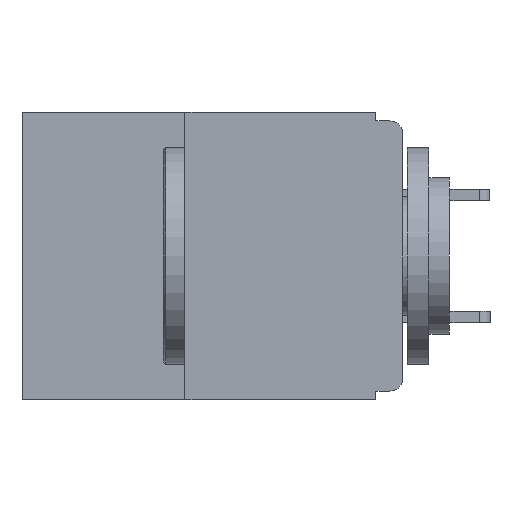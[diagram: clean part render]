
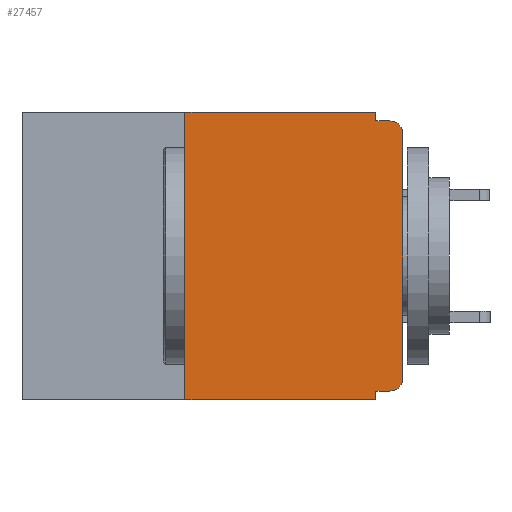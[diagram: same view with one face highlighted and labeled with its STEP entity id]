
A CAD part, left-side view. The second image highlights one B-rep face of the part: STEP entity #27457.
In plain terms, the highlighted planar face has unit normal (-1, 0, 0).
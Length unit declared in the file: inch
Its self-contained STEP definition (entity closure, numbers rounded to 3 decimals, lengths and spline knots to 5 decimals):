
#1856 = ORIENTED_EDGE ( 'NONE', *, *, #5926, .F. ) ;
#2237 = LINE ( 'NONE', #5492, #8270 ) ;
#2534 = CARTESIAN_POINT ( 'NONE',  ( 0., 0.031, -0.33 ) ) ;
#2595 = ORIENTED_EDGE ( 'NONE', *, *, #11031, .F. ) ;
#3029 = ORIENTED_EDGE ( 'NONE', *, *, #3732, .T. ) ;
#3189 = CIRCLE ( 'NONE', #19595, 0.015 ) ;
#3732 = EDGE_CURVE ( 'NONE', #11708, #23164, #3189, .T. ) ;
#4182 = VECTOR ( 'NONE', #6975, 39.37008 ) ;
#5186 = EDGE_CURVE ( 'NONE', #17108, #11934, #23696, .T. ) ;
#5492 = CARTESIAN_POINT ( 'NONE',  ( 0., 0.437, -0.33 ) ) ;
#5926 = EDGE_CURVE ( 'NONE', #29202, #24118, #17416, .T. ) ;
#6591 = PLANE ( 'NONE',  #20163 ) ;
#6975 = DIRECTION ( 'NONE',  ( 0., 0., -1. ) ) ;
#7290 = VERTEX_POINT ( 'NONE', #11916 ) ;
#7435 = EDGE_CURVE ( 'NONE', #14419, #11934, #23615, .T. ) ;
#7765 = CARTESIAN_POINT ( 'NONE',  ( 0., 0., -0.01 ) ) ;
#7867 = DIRECTION ( 'NONE',  ( 0., -1., 0. ) ) ;
#7897 = VERTEX_POINT ( 'NONE', #8672 ) ;
#8225 = ORIENTED_EDGE ( 'NONE', *, *, #27355, .F. ) ;
#8270 = VECTOR ( 'NONE', #14558, 39.37008 ) ;
#8415 = ORIENTED_EDGE ( 'NONE', *, *, #14493, .T. ) ;
#8672 = CARTESIAN_POINT ( 'NONE',  ( 0., 0.25, -0.33 ) ) ;
#8849 = DIRECTION ( 'NONE',  ( 1., 0., 0. ) ) ;
#9213 = CARTESIAN_POINT ( 'NONE',  ( 0., 0.031, 0. ) ) ;
#9583 = ORIENTED_EDGE ( 'NONE', *, *, #5186, .T. ) ;
#10582 = ORIENTED_EDGE ( 'NONE', *, *, #24138, .T. ) ;
#10684 = CARTESIAN_POINT ( 'NONE',  ( 0., 0., -0.32 ) ) ;
#10796 = DIRECTION ( 'NONE',  ( 0., 0., 1. ) ) ;
#11031 = EDGE_CURVE ( 'NONE', #11708, #29202, #25164, .T. ) ;
#11708 = VERTEX_POINT ( 'NONE', #15775 ) ;
#11916 = CARTESIAN_POINT ( 'NONE',  ( 0., 0.25, 0. ) ) ;
#11934 = VERTEX_POINT ( 'NONE', #27694 ) ;
#11983 = LINE ( 'NONE', #27381, #28444 ) ;
#12973 = DIRECTION ( 'NONE',  ( 0., 1., 0. ) ) ;
#13116 = CARTESIAN_POINT ( 'NONE',  ( 0., 0., -0.025 ) ) ;
#13993 = ORIENTED_EDGE ( 'NONE', *, *, #18505, .F. ) ;
#14419 = VERTEX_POINT ( 'NONE', #25546 ) ;
#14493 = EDGE_CURVE ( 'NONE', #7897, #24118, #2237, .T. ) ;
#14558 = DIRECTION ( 'NONE',  ( 0., -1., 0. ) ) ;
#15058 = FACE_OUTER_BOUND ( 'NONE', #21268, .T. ) ;
#15775 = CARTESIAN_POINT ( 'NONE',  ( 0., 0.015, -0.32 ) ) ;
#17108 = VERTEX_POINT ( 'NONE', #13116 ) ;
#17137 = VECTOR ( 'NONE', #12973, 39.37008 ) ;
#17209 = VECTOR ( 'NONE', #10796, 39.37008 ) ;
#17416 = LINE ( 'NONE', #21441, #24051 ) ;
#17811 = CARTESIAN_POINT ( 'NONE',  ( 0., 0.031, -0.32 ) ) ;
#18505 = EDGE_CURVE ( 'NONE', #7290, #25681, #21759, .T. ) ;
#19595 = AXIS2_PLACEMENT_3D ( 'NONE', #25613, #25484, #25479 ) ;
#19777 = ORIENTED_EDGE ( 'NONE', *, *, #7435, .F. ) ;
#20163 = AXIS2_PLACEMENT_3D ( 'NONE', #22416, #8849, #24716 ) ;
#20329 = CARTESIAN_POINT ( 'NONE',  ( 0., 0.437, 0. ) ) ;
#20874 = DIRECTION ( 'NONE',  ( 0., 0., 1. ) ) ;
#20897 = EDGE_CURVE ( 'NONE', #25681, #14419, #22336, .T. ) ;
#21016 = DIRECTION ( 'NONE',  ( -1., 0., 0. ) ) ;
#21242 = DIRECTION ( 'NONE',  ( 0., 0., -1. ) ) ;
#21248 = DIRECTION ( 'NONE',  ( 0., 0., -1. ) ) ;
#21268 = EDGE_LOOP ( 'NONE', ( #10582, #9583, #19777, #22824, #13993, #8225, #8415, #1856, #2595, #3029 ) ) ;
#21275 = CARTESIAN_POINT ( 'NONE',  ( 0., 0.015, -0.025 ) ) ;
#21441 = CARTESIAN_POINT ( 'NONE',  ( 0., 0.031, -0.33 ) ) ;
#21518 = CARTESIAN_POINT ( 'NONE',  ( 0., 0., -0.305 ) ) ;
#21759 = LINE ( 'NONE', #20329, #26871 ) ;
#22336 = LINE ( 'NONE', #9213, #4182 ) ;
#22416 = CARTESIAN_POINT ( 'NONE',  ( 0., 0.437, 0. ) ) ;
#22572 = DIRECTION ( 'NONE',  ( 0., -1., 0. ) ) ;
#22810 = CARTESIAN_POINT ( 'NONE',  ( 0., 0.031, 0. ) ) ;
#22824 = ORIENTED_EDGE ( 'NONE', *, *, #20897, .F. ) ;
#22942 = VECTOR ( 'NONE', #7867, 39.37008 ) ;
#23164 = VERTEX_POINT ( 'NONE', #21518 ) ;
#23166 = LINE ( 'NONE', #24346, #17209 ) ;
#23615 = LINE ( 'NONE', #7765, #22942 ) ;
#23696 = CIRCLE ( 'NONE', #24272, 0.015 ) ;
#24051 = VECTOR ( 'NONE', #21248, 39.37008 ) ;
#24118 = VERTEX_POINT ( 'NONE', #2534 ) ;
#24138 = EDGE_CURVE ( 'NONE', #23164, #17108, #11983, .T. ) ;
#24272 = AXIS2_PLACEMENT_3D ( 'NONE', #21275, #21016, #21242 ) ;
#24346 = CARTESIAN_POINT ( 'NONE',  ( 0., 0.25, -0.33 ) ) ;
#24716 = DIRECTION ( 'NONE',  ( 0., 0., -1. ) ) ;
#25164 = LINE ( 'NONE', #10684, #17137 ) ;
#25479 = DIRECTION ( 'NONE',  ( 0., 0., -1. ) ) ;
#25484 = DIRECTION ( 'NONE',  ( -1., 0., 0. ) ) ;
#25546 = CARTESIAN_POINT ( 'NONE',  ( 0., 0.031, -0.01 ) ) ;
#25613 = CARTESIAN_POINT ( 'NONE',  ( 0., 0.015, -0.305 ) ) ;
#25681 = VERTEX_POINT ( 'NONE', #22810 ) ;
#26871 = VECTOR ( 'NONE', #22572, 39.37008 ) ;
#27355 = EDGE_CURVE ( 'NONE', #7897, #7290, #23166, .T. ) ;
#27381 = CARTESIAN_POINT ( 'NONE',  ( 0., 0., 0. ) ) ;
#27457 = ADVANCED_FACE ( 'NONE', ( #15058 ), #6591, .F. ) ;
#27694 = CARTESIAN_POINT ( 'NONE',  ( 0., 0.015, -0.01 ) ) ;
#28444 = VECTOR ( 'NONE', #20874, 39.37008 ) ;
#29202 = VERTEX_POINT ( 'NONE', #17811 ) ;
